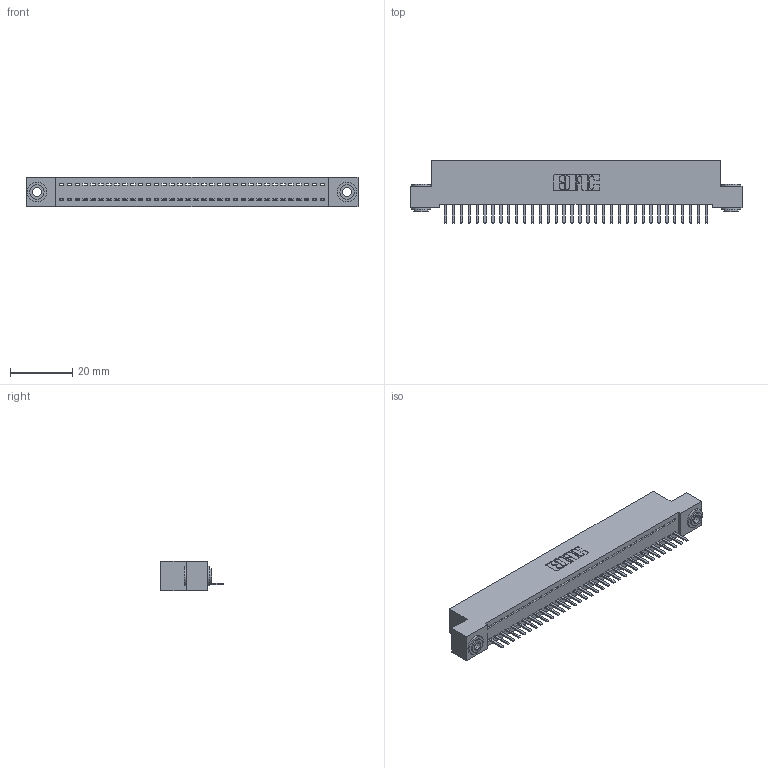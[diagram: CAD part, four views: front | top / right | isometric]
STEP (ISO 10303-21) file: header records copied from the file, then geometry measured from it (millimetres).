
FILE_DESCRIPTION (( 'STEP AP203' ), '1' );
FILE_NAME ('342-034-520-103.STEP', '2018-08-11T18:08:16', ( '' ), ( '' ), 'SwSTEP 2.0', 'SolidWorks 2016', '' );
FILE_SCHEMA (( 'CONFIG_CONTROL_DESIGN' ));
Length unit declared in the file: inch
Products named in the file (4): 342 Part_.156 TH; 345-292-001_345-293-120; 342-250-002_345-250-002-102; 342-034-520-103
Assembly tree (37 placements, depth 2):
  342-034-520-103
    342 Part_.156 TH
    345-292-001_345-293-120  x34
    342-250-002_345-250-002-102  x2
Bounding box: 106.68 x 20.02 x 9.4 mm (x, y, z)
Volume: 9249.3 mm3; surface area: 13346.1 mm2
Topology: 37 solids, 37 shells, 2256 faces, 6631 edges, 4326 vertices
Faces by surface type: plane 1572, cylinder 676, cone 8
Entity records: 22452 total; most frequent: CARTESIAN_POINT 3863, ORIENTED_EDGE 3814, DIRECTION 3297, EDGE_CURVE 1907, VECTOR 1751, LINE 1751, VERTEX_POINT 1266, AXIS2_PLACEMENT_3D 773
